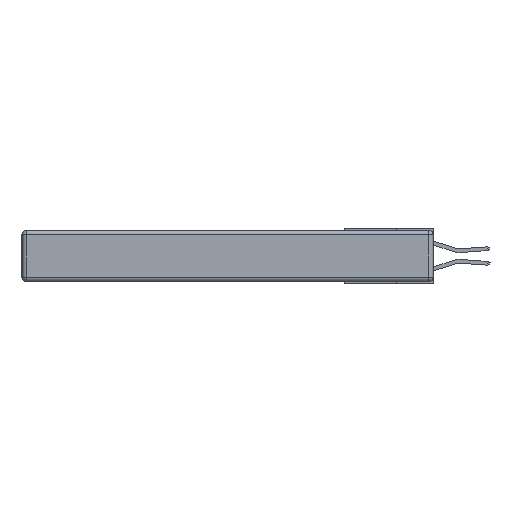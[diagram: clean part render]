
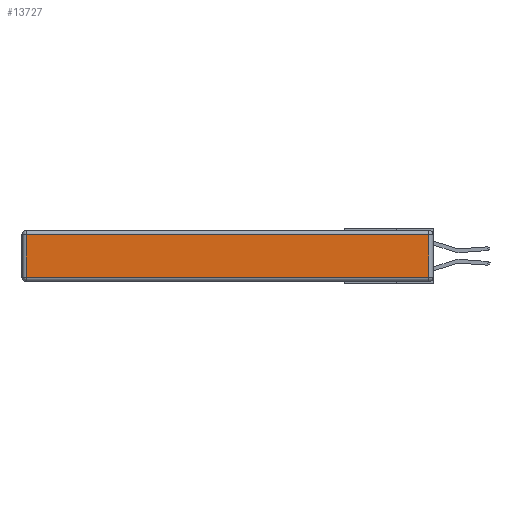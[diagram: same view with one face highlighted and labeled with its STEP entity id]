
A CAD part, left-side view. The second image highlights one B-rep face of the part: STEP entity #13727.
In plain terms, the highlighted planar face has unit normal (-1, 0, 0).
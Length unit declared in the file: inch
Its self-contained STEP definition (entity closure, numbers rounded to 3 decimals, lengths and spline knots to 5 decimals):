
#852 = DIRECTION ( 'NONE',  ( 0., -1., 0. ) ) ;
#1546 = CARTESIAN_POINT ( 'NONE',  ( 0., 2.72, -0.343 ) ) ;
#2155 = ORIENTED_EDGE ( 'NONE', *, *, #14699, .T. ) ;
#2502 = EDGE_CURVE ( 'NONE', #3693, #18711, #3834, .T. ) ;
#3133 = PLANE ( 'NONE',  #15416 ) ;
#3490 = LINE ( 'NONE', #4844, #6120 ) ;
#3693 = VERTEX_POINT ( 'NONE', #18118 ) ;
#3834 = LINE ( 'NONE', #1546, #6945 ) ;
#3981 = EDGE_LOOP ( 'NONE', ( #2155, #16491, #13719, #16334 ) ) ;
#4306 = VECTOR ( 'NONE', #852, 39.37008 ) ;
#4800 = CARTESIAN_POINT ( 'NONE',  ( 0., 0., -0.343 ) ) ;
#4844 = CARTESIAN_POINT ( 'NONE',  ( 0., 2.75, -0.03 ) ) ;
#6074 = DIRECTION ( 'NONE',  ( -1., 0., 0. ) ) ;
#6120 = VECTOR ( 'NONE', #14219, 39.37008 ) ;
#6166 = DIRECTION ( 'NONE',  ( 0., 0., -1. ) ) ;
#6945 = VECTOR ( 'NONE', #6166, 39.37008 ) ;
#7015 = CARTESIAN_POINT ( 'NONE',  ( 0., 0.03, -0.313 ) ) ;
#7267 = CARTESIAN_POINT ( 'NONE',  ( 0., 2.72, -0.313 ) ) ;
#8573 = VERTEX_POINT ( 'NONE', #11316 ) ;
#9358 = LINE ( 'NONE', #11506, #4306 ) ;
#10917 = EDGE_CURVE ( 'NONE', #8573, #3693, #3490, .T. ) ;
#11316 = CARTESIAN_POINT ( 'NONE',  ( 0., 0.03, -0.03 ) ) ;
#11506 = CARTESIAN_POINT ( 'NONE',  ( 0., 0., -0.313 ) ) ;
#11810 = CARTESIAN_POINT ( 'NONE',  ( 0., 0.03, -0.343 ) ) ;
#12327 = FACE_OUTER_BOUND ( 'NONE', #3981, .T. ) ;
#13068 = VECTOR ( 'NONE', #16187, 39.37008 ) ;
#13393 = EDGE_CURVE ( 'NONE', #18008, #8573, #17835, .T. ) ;
#13719 = ORIENTED_EDGE ( 'NONE', *, *, #10917, .T. ) ;
#13727 = ADVANCED_FACE ( 'NONE', ( #12327 ), #3133, .T. ) ;
#14219 = DIRECTION ( 'NONE',  ( 0., 1., 0. ) ) ;
#14699 = EDGE_CURVE ( 'NONE', #18711, #18008, #9358, .T. ) ;
#15416 = AXIS2_PLACEMENT_3D ( 'NONE', #4800, #6074, #17054 ) ;
#16187 = DIRECTION ( 'NONE',  ( 0., 0., 1. ) ) ;
#16334 = ORIENTED_EDGE ( 'NONE', *, *, #2502, .T. ) ;
#16491 = ORIENTED_EDGE ( 'NONE', *, *, #13393, .T. ) ;
#17054 = DIRECTION ( 'NONE',  ( 0., 0., 1. ) ) ;
#17835 = LINE ( 'NONE', #11810, #13068 ) ;
#18008 = VERTEX_POINT ( 'NONE', #7015 ) ;
#18118 = CARTESIAN_POINT ( 'NONE',  ( 0., 2.72, -0.03 ) ) ;
#18711 = VERTEX_POINT ( 'NONE', #7267 ) ;
